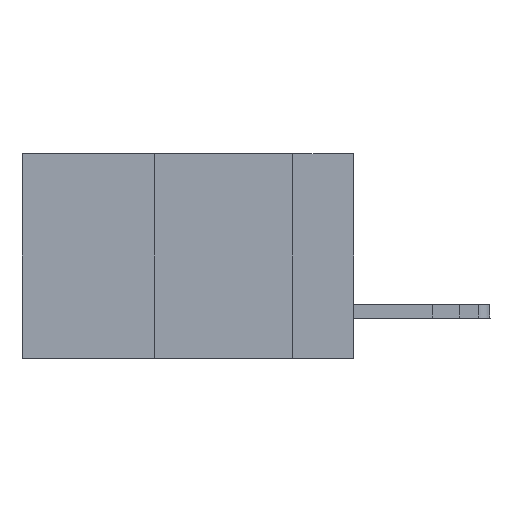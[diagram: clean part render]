
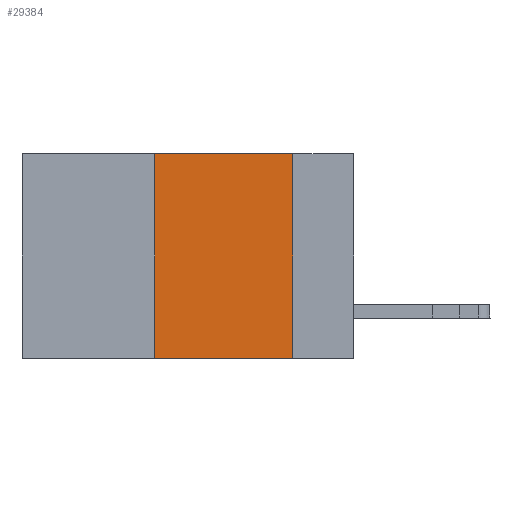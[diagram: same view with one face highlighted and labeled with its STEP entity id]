
A CAD part, left-side view. The second image highlights one B-rep face of the part: STEP entity #29384.
In plain terms, the highlighted planar face has unit normal (-1, 0, 0).
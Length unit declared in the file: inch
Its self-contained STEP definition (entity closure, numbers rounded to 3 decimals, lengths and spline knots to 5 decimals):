
#442 = CARTESIAN_POINT ( 'NONE',  ( 0., 0.6, -0.37 ) ) ;
#496 = VECTOR ( 'NONE', #8352, 39.37008 ) ;
#1758 = PLANE ( 'NONE',  #18671 ) ;
#2535 = VERTEX_POINT ( 'NONE', #19987 ) ;
#5922 = ORIENTED_EDGE ( 'NONE', *, *, #32069, .F. ) ;
#6642 = EDGE_CURVE ( 'NONE', #12822, #2535, #19299, .T. ) ;
#8352 = DIRECTION ( 'NONE',  ( 0., -1., 0. ) ) ;
#9626 = ORIENTED_EDGE ( 'NONE', *, *, #6642, .T. ) ;
#11763 = VECTOR ( 'NONE', #12317, 39.37008 ) ;
#12317 = DIRECTION ( 'NONE',  ( 0., 0., 1. ) ) ;
#12822 = VERTEX_POINT ( 'NONE', #17269 ) ;
#12985 = CARTESIAN_POINT ( 'NONE',  ( 0., 0.6, 0. ) ) ;
#13651 = LINE ( 'NONE', #12985, #496 ) ;
#14526 = EDGE_CURVE ( 'NONE', #12822, #31411, #19448, .T. ) ;
#14744 = VECTOR ( 'NONE', #27900, 39.37008 ) ;
#16049 = DIRECTION ( 'NONE',  ( 0., 0., -1. ) ) ;
#16333 = EDGE_LOOP ( 'NONE', ( #21252, #5922, #35359, #9626 ) ) ;
#17269 = CARTESIAN_POINT ( 'NONE',  ( 0., 0.36, -0.37 ) ) ;
#17604 = CARTESIAN_POINT ( 'NONE',  ( 0., 0.36, 0. ) ) ;
#18671 = AXIS2_PLACEMENT_3D ( 'NONE', #33526, #30494, #16049 ) ;
#19299 = LINE ( 'NONE', #442, #29578 ) ;
#19448 = LINE ( 'NONE', #29528, #11763 ) ;
#19987 = CARTESIAN_POINT ( 'NONE',  ( 0., 0.11, -0.37 ) ) ;
#20179 = FACE_OUTER_BOUND ( 'NONE', #16333, .T. ) ;
#20450 = DIRECTION ( 'NONE',  ( 0., -1., 0. ) ) ;
#20555 = VERTEX_POINT ( 'NONE', #30718 ) ;
#21252 = ORIENTED_EDGE ( 'NONE', *, *, #28902, .F. ) ;
#27775 = CARTESIAN_POINT ( 'NONE',  ( 0., 0.11, 0. ) ) ;
#27900 = DIRECTION ( 'NONE',  ( 0., 0., -1. ) ) ;
#28902 = EDGE_CURVE ( 'NONE', #20555, #2535, #32774, .T. ) ;
#29384 = ADVANCED_FACE ( 'NONE', ( #20179 ), #1758, .F. ) ;
#29528 = CARTESIAN_POINT ( 'NONE',  ( 0., 0.36, 0. ) ) ;
#29578 = VECTOR ( 'NONE', #20450, 39.37008 ) ;
#30494 = DIRECTION ( 'NONE',  ( 1., 0., 0. ) ) ;
#30718 = CARTESIAN_POINT ( 'NONE',  ( 0., 0.11, 0. ) ) ;
#31411 = VERTEX_POINT ( 'NONE', #17604 ) ;
#32069 = EDGE_CURVE ( 'NONE', #31411, #20555, #13651, .T. ) ;
#32774 = LINE ( 'NONE', #27775, #14744 ) ;
#33526 = CARTESIAN_POINT ( 'NONE',  ( 0., 0.6, 0. ) ) ;
#35359 = ORIENTED_EDGE ( 'NONE', *, *, #14526, .F. ) ;
